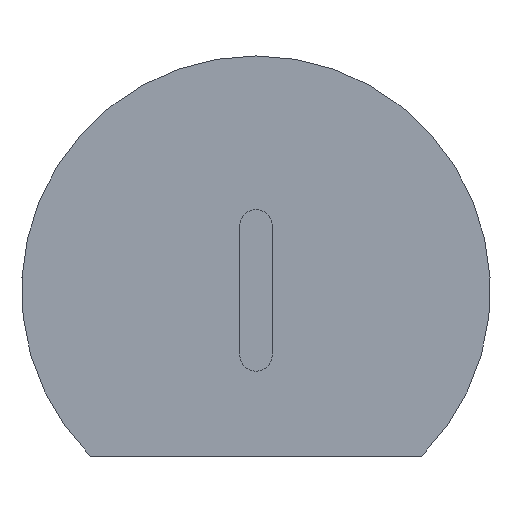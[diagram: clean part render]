
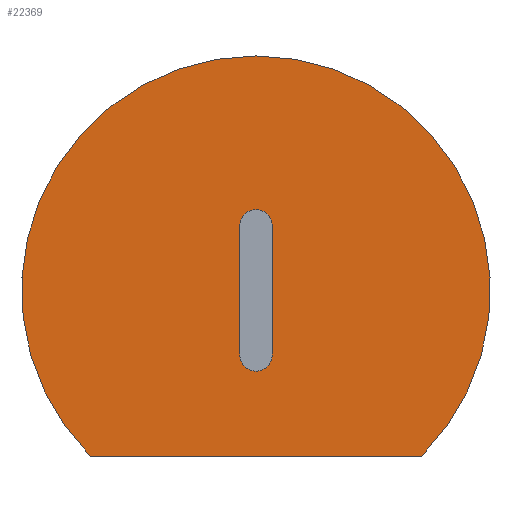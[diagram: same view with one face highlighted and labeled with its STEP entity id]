
A CAD part, left-side view. The second image highlights one B-rep face of the part: STEP entity #22369.
In plain terms, the highlighted planar face has unit normal (-1, 0, 0).
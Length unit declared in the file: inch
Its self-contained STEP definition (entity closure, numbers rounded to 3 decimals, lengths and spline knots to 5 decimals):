
#411 = DIRECTION ( 'NONE',  ( 0., 0., 1. ) ) ;
#948 = CARTESIAN_POINT ( 'NONE',  ( -0.75, 0.95512, -0.205 ) ) ;
#1035 = CARTESIAN_POINT ( 'NONE',  ( -0.75, 0.75, 0.1 ) ) ;
#1100 = ORIENTED_EDGE ( 'NONE', *, *, #1744, .T. ) ;
#1478 = DIRECTION ( 'NONE',  ( -1., 0., 0. ) ) ;
#1627 = CARTESIAN_POINT ( 'NONE',  ( -0.75, 0.73, 0.08 ) ) ;
#1744 = EDGE_CURVE ( 'NONE', #16239, #13106, #8012, .T. ) ;
#1778 = ORIENTED_EDGE ( 'NONE', *, *, #22098, .F. ) ;
#1997 = FACE_BOUND ( 'NONE', #18076, .T. ) ;
#3111 = CARTESIAN_POINT ( 'NONE',  ( -0.75, 1.05, -0.205 ) ) ;
#3161 = AXIS2_PLACEMENT_3D ( 'NONE', #14087, #3225, #10526 ) ;
#3225 = DIRECTION ( 'NONE',  ( -1., 0., 0. ) ) ;
#4294 = VECTOR ( 'NONE', #8425, 39.37008 ) ;
#4903 = VERTEX_POINT ( 'NONE', #19431 ) ;
#5419 = CIRCLE ( 'NONE', #7554, 0.02 ) ;
#5646 = EDGE_CURVE ( 'NONE', #4903, #6127, #10796, .T. ) ;
#5973 = VECTOR ( 'NONE', #12589, 39.37008 ) ;
#6127 = VERTEX_POINT ( 'NONE', #12389 ) ;
#6661 = ORIENTED_EDGE ( 'NONE', *, *, #15851, .T. ) ;
#6876 = CARTESIAN_POINT ( 'NONE',  ( -0.75, 0.75, 0. ) ) ;
#7554 = AXIS2_PLACEMENT_3D ( 'NONE', #14156, #17951, #15990 ) ;
#7639 = DIRECTION ( 'NONE',  ( -1., 0., 0. ) ) ;
#7986 = LINE ( 'NONE', #3111, #4294 ) ;
#8012 = CIRCLE ( 'NONE', #19068, 0.29 ) ;
#8257 = FACE_OUTER_BOUND ( 'NONE', #13205, .T. ) ;
#8425 = DIRECTION ( 'NONE',  ( 0., -1., 0. ) ) ;
#8456 = PLANE ( 'NONE',  #8779 ) ;
#8473 = DIRECTION ( 'NONE',  ( 0., 0., 1. ) ) ;
#8779 = AXIS2_PLACEMENT_3D ( 'NONE', #6876, #10296, #10451 ) ;
#8812 = LINE ( 'NONE', #10523, #15926 ) ;
#9446 = DIRECTION ( 'NONE',  ( -1., 0., 0. ) ) ;
#10296 = DIRECTION ( 'NONE',  ( -1., 0., 0. ) ) ;
#10451 = DIRECTION ( 'NONE',  ( 0., 0., 1. ) ) ;
#10523 = CARTESIAN_POINT ( 'NONE',  ( -0.75, 0.73, -0.08 ) ) ;
#10526 = DIRECTION ( 'NONE',  ( 0., 0., 1. ) ) ;
#10732 = CIRCLE ( 'NONE', #13399, 0.29 ) ;
#10796 = LINE ( 'NONE', #10928, #5973 ) ;
#10928 = CARTESIAN_POINT ( 'NONE',  ( -0.75, 0.77, -0.08 ) ) ;
#11795 = VERTEX_POINT ( 'NONE', #1627 ) ;
#12341 = CARTESIAN_POINT ( 'NONE',  ( -0.75, 0.73, -0.08 ) ) ;
#12389 = CARTESIAN_POINT ( 'NONE',  ( -0.75, 0.77, -0.08 ) ) ;
#12589 = DIRECTION ( 'NONE',  ( 0., 0., -1. ) ) ;
#12856 = VERTEX_POINT ( 'NONE', #948 ) ;
#13104 = DIRECTION ( 'NONE',  ( 0., 0., 1. ) ) ;
#13106 = VERTEX_POINT ( 'NONE', #21050 ) ;
#13205 = EDGE_LOOP ( 'NONE', ( #14821, #1100, #6661 ) ) ;
#13270 = CARTESIAN_POINT ( 'NONE',  ( -0.75, 0.75, 0. ) ) ;
#13399 = AXIS2_PLACEMENT_3D ( 'NONE', #16749, #9446, #411 ) ;
#14087 = CARTESIAN_POINT ( 'NONE',  ( -0.75, 0.75, 0.08 ) ) ;
#14156 = CARTESIAN_POINT ( 'NONE',  ( -0.75, 0.75, -0.08 ) ) ;
#14821 = ORIENTED_EDGE ( 'NONE', *, *, #22574, .T. ) ;
#14971 = ORIENTED_EDGE ( 'NONE', *, *, #23319, .F. ) ;
#15695 = ORIENTED_EDGE ( 'NONE', *, *, #17673, .F. ) ;
#15851 = EDGE_CURVE ( 'NONE', #13106, #12856, #10732, .T. ) ;
#15926 = VECTOR ( 'NONE', #23194, 39.37008 ) ;
#15990 = DIRECTION ( 'NONE',  ( 0., 0., 1. ) ) ;
#16239 = VERTEX_POINT ( 'NONE', #20796 ) ;
#16749 = CARTESIAN_POINT ( 'NONE',  ( -0.75, 0.75, 0. ) ) ;
#17083 = AXIS2_PLACEMENT_3D ( 'NONE', #19501, #1478, #8473 ) ;
#17224 = VERTEX_POINT ( 'NONE', #1035 ) ;
#17355 = CIRCLE ( 'NONE', #3161, 0.02 ) ;
#17673 = EDGE_CURVE ( 'NONE', #11795, #17224, #21551, .T. ) ;
#17951 = DIRECTION ( 'NONE',  ( -1., 0., 0. ) ) ;
#18076 = EDGE_LOOP ( 'NONE', ( #18165, #20594, #1778, #15695, #14971 ) ) ;
#18165 = ORIENTED_EDGE ( 'NONE', *, *, #21657, .F. ) ;
#19068 = AXIS2_PLACEMENT_3D ( 'NONE', #13270, #7639, #13104 ) ;
#19431 = CARTESIAN_POINT ( 'NONE',  ( -0.75, 0.77, 0.08 ) ) ;
#19501 = CARTESIAN_POINT ( 'NONE',  ( -0.75, 0.75, 0.08 ) ) ;
#20594 = ORIENTED_EDGE ( 'NONE', *, *, #5646, .F. ) ;
#20796 = CARTESIAN_POINT ( 'NONE',  ( -0.75, 0.54488, -0.205 ) ) ;
#21050 = CARTESIAN_POINT ( 'NONE',  ( -0.75, 0.75, 0.29 ) ) ;
#21551 = CIRCLE ( 'NONE', #17083, 0.02 ) ;
#21657 = EDGE_CURVE ( 'NONE', #6127, #22212, #5419, .T. ) ;
#22098 = EDGE_CURVE ( 'NONE', #17224, #4903, #17355, .T. ) ;
#22212 = VERTEX_POINT ( 'NONE', #12341 ) ;
#22369 = ADVANCED_FACE ( 'NONE', ( #1997, #8257 ), #8456, .T. ) ;
#22574 = EDGE_CURVE ( 'NONE', #12856, #16239, #7986, .T. ) ;
#23194 = DIRECTION ( 'NONE',  ( 0., 0., 1. ) ) ;
#23319 = EDGE_CURVE ( 'NONE', #22212, #11795, #8812, .T. ) ;
